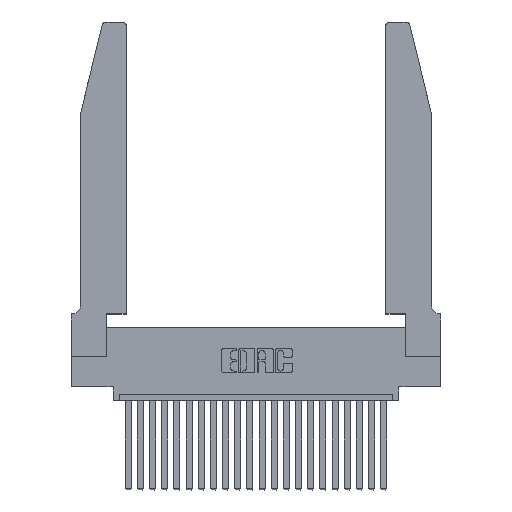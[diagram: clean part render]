
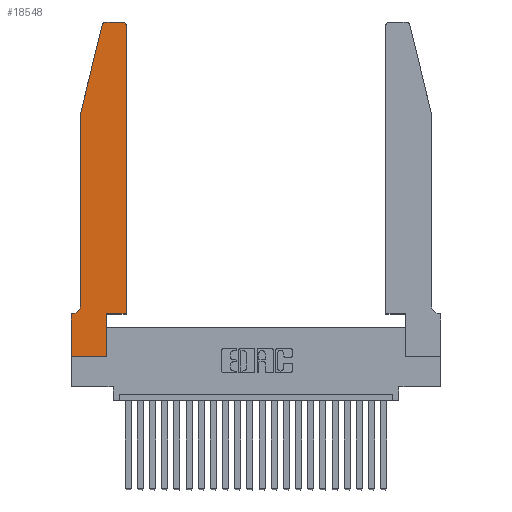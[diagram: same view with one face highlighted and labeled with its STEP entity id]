
A CAD part, top view. The second image highlights one B-rep face of the part: STEP entity #18548.
In plain terms, the highlighted planar face has unit normal (0, 0, 1).
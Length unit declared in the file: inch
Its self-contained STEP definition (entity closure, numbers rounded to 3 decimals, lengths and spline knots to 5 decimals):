
#71 = CARTESIAN_POINT ( 'NONE',  ( 0.0755, 2., 0.37 ) ) ;
#306 = VECTOR ( 'NONE', #22501, 39.37008 ) ;
#516 = CARTESIAN_POINT ( 'NONE',  ( 0.4505, 0.35, 0.37 ) ) ;
#520 = VECTOR ( 'NONE', #6147, 39.37008 ) ;
#577 = VECTOR ( 'NONE', #11357, 39.37008 ) ;
#589 = CARTESIAN_POINT ( 'NONE',  ( 0.2865, 0.35, 0.37 ) ) ;
#727 = EDGE_LOOP ( 'NONE', ( #13319, #21816, #12774, #2463, #4003, #14623, #2540, #13861, #19192, #4063, #4809, #22557 ) ) ;
#754 = VERTEX_POINT ( 'NONE', #11095 ) ;
#902 = AXIS2_PLACEMENT_3D ( 'NONE', #23463, #12433, #11062 ) ;
#916 = VECTOR ( 'NONE', #12976, 39.37008 ) ;
#1364 = EDGE_CURVE ( 'NONE', #22872, #13630, #7912, .T. ) ;
#1829 = EDGE_CURVE ( 'NONE', #22611, #3338, #17708, .T. ) ;
#2078 = CARTESIAN_POINT ( 'NONE',  ( 0.0755, 2., 0.37 ) ) ;
#2269 = CIRCLE ( 'NONE', #18858, 0.03 ) ;
#2463 = ORIENTED_EDGE ( 'NONE', *, *, #10437, .T. ) ;
#2540 = ORIENTED_EDGE ( 'NONE', *, *, #5773, .T. ) ;
#3050 = EDGE_CURVE ( 'NONE', #14099, #22611, #4076, .T. ) ;
#3338 = VERTEX_POINT ( 'NONE', #589 ) ;
#3768 = DIRECTION ( 'NONE',  ( 0., 1., 0. ) ) ;
#3873 = PLANE ( 'NONE',  #4348 ) ;
#4003 = ORIENTED_EDGE ( 'NONE', *, *, #21773, .T. ) ;
#4046 = DIRECTION ( 'NONE',  ( -1., 0., 0. ) ) ;
#4063 = ORIENTED_EDGE ( 'NONE', *, *, #18230, .T. ) ;
#4076 = LINE ( 'NONE', #6443, #520 ) ;
#4348 = AXIS2_PLACEMENT_3D ( 'NONE', #16786, #5749, #7578 ) ;
#4809 = ORIENTED_EDGE ( 'NONE', *, *, #18729, .T. ) ;
#5013 = VECTOR ( 'NONE', #3768, 39.37008 ) ;
#5035 = LINE ( 'NONE', #516, #7325 ) ;
#5088 = DIRECTION ( 'NONE',  ( -1., 0., 0. ) ) ;
#5165 = AXIS2_PLACEMENT_3D ( 'NONE', #11364, #11284, #7723 ) ;
#5749 = DIRECTION ( 'NONE',  ( 0., 0., 1. ) ) ;
#5773 = EDGE_CURVE ( 'NONE', #13630, #14099, #15125, .T. ) ;
#6147 = DIRECTION ( 'NONE',  ( 1., 0., 0. ) ) ;
#6235 = EDGE_CURVE ( 'NONE', #7626, #19359, #9305, .T. ) ;
#6443 = CARTESIAN_POINT ( 'NONE',  ( 0., 0., 0.37 ) ) ;
#6952 = CARTESIAN_POINT ( 'NONE',  ( 0.4505, 0.35, 0.37 ) ) ;
#6973 = CARTESIAN_POINT ( 'NONE',  ( 0.4205, 2.72, 0.37 ) ) ;
#7321 = CARTESIAN_POINT ( 'NONE',  ( 0.0055, 0.35, 0.37 ) ) ;
#7325 = VECTOR ( 'NONE', #15375, 39.37008 ) ;
#7578 = DIRECTION ( 'NONE',  ( 1., 0., 0. ) ) ;
#7624 = FACE_OUTER_BOUND ( 'NONE', #727, .T. ) ;
#7626 = VERTEX_POINT ( 'NONE', #11185 ) ;
#7723 = DIRECTION ( 'NONE',  ( -1., 0., 0. ) ) ;
#7912 = LINE ( 'NONE', #9366, #21457 ) ;
#7941 = VECTOR ( 'NONE', #21853, 39.37008 ) ;
#8633 = CARTESIAN_POINT ( 'NONE',  ( 0., 0.35, 0.37 ) ) ;
#8751 = LINE ( 'NONE', #13135, #5013 ) ;
#9294 = EDGE_CURVE ( 'NONE', #17459, #15958, #21260, .T. ) ;
#9305 = LINE ( 'NONE', #71, #577 ) ;
#9366 = CARTESIAN_POINT ( 'NONE',  ( 0.0755, 0.35, 0.37 ) ) ;
#9540 = CARTESIAN_POINT ( 'NONE',  ( 0.2865, 0.35, 0.37 ) ) ;
#9797 = CARTESIAN_POINT ( 'NONE',  ( 0., 0., 0.37 ) ) ;
#10437 = EDGE_CURVE ( 'NONE', #19359, #754, #17473, .T. ) ;
#11062 = DIRECTION ( 'NONE',  ( 1., 0., 0. ) ) ;
#11095 = CARTESIAN_POINT ( 'NONE',  ( 0.0755, 0.42, 0.37 ) ) ;
#11185 = CARTESIAN_POINT ( 'NONE',  ( 0.25487, 2.72718, 0.37 ) ) ;
#11255 = VERTEX_POINT ( 'NONE', #17538 ) ;
#11284 = DIRECTION ( 'NONE',  ( 0., 0., -1. ) ) ;
#11357 = DIRECTION ( 'NONE',  ( -0.239, -0.971, 0. ) ) ;
#11364 = CARTESIAN_POINT ( 'NONE',  ( 0.0055, 0.42, 0.37 ) ) ;
#11547 = CARTESIAN_POINT ( 'NONE',  ( 0., 0., 0.37 ) ) ;
#12433 = DIRECTION ( 'NONE',  ( 0., 0., 1. ) ) ;
#12774 = ORIENTED_EDGE ( 'NONE', *, *, #6235, .T. ) ;
#12976 = DIRECTION ( 'NONE',  ( 0., -1., 0. ) ) ;
#13135 = CARTESIAN_POINT ( 'NONE',  ( 0.4505, 0.35, 0.37 ) ) ;
#13319 = ORIENTED_EDGE ( 'NONE', *, *, #9294, .T. ) ;
#13630 = VERTEX_POINT ( 'NONE', #8633 ) ;
#13861 = ORIENTED_EDGE ( 'NONE', *, *, #3050, .T. ) ;
#14099 = VERTEX_POINT ( 'NONE', #11547 ) ;
#14195 = CARTESIAN_POINT ( 'NONE',  ( 0.4205, 2.75, 0.37 ) ) ;
#14498 = EDGE_CURVE ( 'NONE', #11255, #17459, #2269, .T. ) ;
#14623 = ORIENTED_EDGE ( 'NONE', *, *, #1364, .T. ) ;
#15125 = LINE ( 'NONE', #9797, #916 ) ;
#15261 = CIRCLE ( 'NONE', #5165, 0.07 ) ;
#15375 = DIRECTION ( 'NONE',  ( 1., 0., 0. ) ) ;
#15911 = CARTESIAN_POINT ( 'NONE',  ( 0.2865, 0., 0.37 ) ) ;
#15958 = VERTEX_POINT ( 'NONE', #20204 ) ;
#16023 = DIRECTION ( 'NONE',  ( 1., 0., 0. ) ) ;
#16786 = CARTESIAN_POINT ( 'NONE',  ( 0., 0.35, 0.37 ) ) ;
#17459 = VERTEX_POINT ( 'NONE', #14195 ) ;
#17466 = CARTESIAN_POINT ( 'NONE',  ( 0.0755, 2., 0.37 ) ) ;
#17473 = LINE ( 'NONE', #17466, #7941 ) ;
#17538 = CARTESIAN_POINT ( 'NONE',  ( 0.4505, 2.72, 0.37 ) ) ;
#17708 = LINE ( 'NONE', #9540, #306 ) ;
#18230 = EDGE_CURVE ( 'NONE', #3338, #20062, #5035, .T. ) ;
#18548 = ADVANCED_FACE ( 'NONE', ( #7624 ), #3873, .T. ) ;
#18687 = EDGE_CURVE ( 'NONE', #15958, #7626, #23464, .T. ) ;
#18729 = EDGE_CURVE ( 'NONE', #20062, #11255, #8751, .T. ) ;
#18858 = AXIS2_PLACEMENT_3D ( 'NONE', #6973, #21567, #16023 ) ;
#19192 = ORIENTED_EDGE ( 'NONE', *, *, #1829, .T. ) ;
#19359 = VERTEX_POINT ( 'NONE', #2078 ) ;
#20062 = VERTEX_POINT ( 'NONE', #6952 ) ;
#20204 = CARTESIAN_POINT ( 'NONE',  ( 0.284, 2.75, 0.37 ) ) ;
#20684 = VECTOR ( 'NONE', #5088, 39.37008 ) ;
#21260 = LINE ( 'NONE', #21608, #20684 ) ;
#21457 = VECTOR ( 'NONE', #4046, 39.37008 ) ;
#21567 = DIRECTION ( 'NONE',  ( 0., 0., 1. ) ) ;
#21608 = CARTESIAN_POINT ( 'NONE',  ( 0.2605, 2.75, 0.37 ) ) ;
#21773 = EDGE_CURVE ( 'NONE', #754, #22872, #15261, .T. ) ;
#21816 = ORIENTED_EDGE ( 'NONE', *, *, #18687, .T. ) ;
#21853 = DIRECTION ( 'NONE',  ( 0., -1., 0. ) ) ;
#22501 = DIRECTION ( 'NONE',  ( 0., 1., 0. ) ) ;
#22557 = ORIENTED_EDGE ( 'NONE', *, *, #14498, .T. ) ;
#22611 = VERTEX_POINT ( 'NONE', #15911 ) ;
#22872 = VERTEX_POINT ( 'NONE', #7321 ) ;
#23463 = CARTESIAN_POINT ( 'NONE',  ( 0.284, 2.72, 0.37 ) ) ;
#23464 = CIRCLE ( 'NONE', #902, 0.03 ) ;
